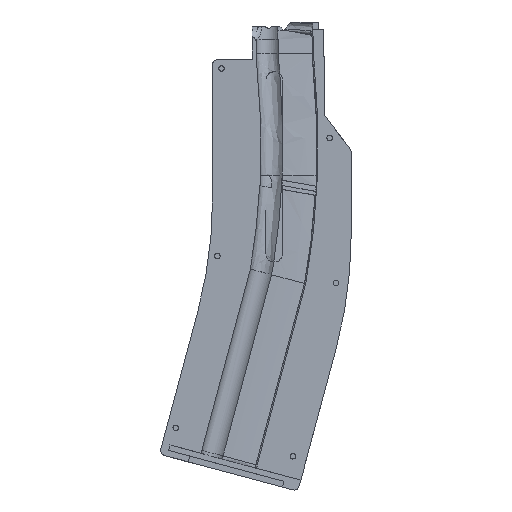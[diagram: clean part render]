
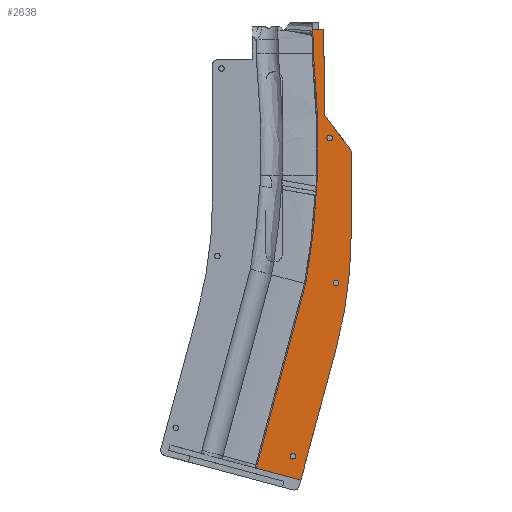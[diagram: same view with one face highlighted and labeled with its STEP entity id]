
A CAD part, front view. The second image highlights one B-rep face of the part: STEP entity #2638.
In plain terms, the highlighted planar face has unit normal (0, -1, 0).
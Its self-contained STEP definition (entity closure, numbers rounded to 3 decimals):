
#15=FACE_BOUND('',#458,.T.);
#16=FACE_BOUND('',#459,.T.);
#17=FACE_BOUND('',#460,.T.);
#39=PLANE('',#2853);
#101=B_SPLINE_CURVE_WITH_KNOTS('',3,(#4024,#4025,#4026,#4027),
 .UNSPECIFIED.,.F.,.F.,(4,4),(-10.66,-5.148),
 .UNSPECIFIED.);
#102=B_SPLINE_CURVE_WITH_KNOTS('',3,(#4029,#4030,#4031,#4032),
 .UNSPECIFIED.,.F.,.F.,(4,4),(-5.148,-0.178),
 .UNSPECIFIED.);
#290=FACE_OUTER_BOUND('',#457,.T.);
#457=EDGE_LOOP('',(#1914,#1915,#1916,#1917,#1918,#1919,#1920,#1921,#1922,
#1923,#1924,#1925,#1926,#1927,#1928,#1929,#1930,#1931,#1932));
#458=EDGE_LOOP('',(#1933));
#459=EDGE_LOOP('',(#1934));
#460=EDGE_LOOP('',(#1935));
#638=CIRCLE('',#2803,3.);
#660=CIRCLE('',#2848,200.);
#662=CIRCLE('',#2851,2.5);
#663=CIRCLE('',#2854,2.);
#664=CIRCLE('',#2855,318.391);
#665=CIRCLE('',#2856,1.25);
#666=CIRCLE('',#2857,1.25);
#667=CIRCLE('',#2858,1.25);
#745=LINE('',#3823,#918);
#759=LINE('',#3877,#932);
#761=LINE('',#3881,#934);
#764=LINE('',#3893,#937);
#782=LINE('',#3943,#955);
#786=LINE('',#3957,#959);
#789=LINE('',#4014,#962);
#790=LINE('',#4016,#963);
#791=LINE('',#4018,#964);
#792=LINE('',#4022,#965);
#793=LINE('',#4034,#966);
#794=LINE('',#4036,#967);
#918=VECTOR('',#3109,10.);
#932=VECTOR('',#3151,10.);
#934=VECTOR('',#3155,10.);
#937=VECTOR('',#3170,10.);
#955=VECTOR('',#3218,10.);
#959=VECTOR('',#3234,10.);
#962=VECTOR('',#3239,10.);
#963=VECTOR('',#3240,10.);
#964=VECTOR('',#3241,10.);
#965=VECTOR('',#3244,10.);
#966=VECTOR('',#3245,10.);
#967=VECTOR('',#3246,10.);
#1088=VERTEX_POINT('',#3800);
#1089=VERTEX_POINT('',#3802);
#1094=VERTEX_POINT('',#3821);
#1111=VERTEX_POINT('',#3875);
#1112=VERTEX_POINT('',#3879);
#1115=VERTEX_POINT('',#3892);
#1131=VERTEX_POINT('',#3940);
#1132=VERTEX_POINT('',#3942);
#1135=VERTEX_POINT('',#3952);
#1136=VERTEX_POINT('',#3956);
#1143=VERTEX_POINT('',#4013);
#1144=VERTEX_POINT('',#4015);
#1145=VERTEX_POINT('',#4017);
#1146=VERTEX_POINT('',#4019);
#1147=VERTEX_POINT('',#4021);
#1148=VERTEX_POINT('',#4023);
#1149=VERTEX_POINT('',#4028);
#1150=VERTEX_POINT('',#4033);
#1151=VERTEX_POINT('',#4035);
#1152=VERTEX_POINT('',#4038);
#1153=VERTEX_POINT('',#4040);
#1154=VERTEX_POINT('',#4042);
#1350=EDGE_CURVE('',#1088,#1089,#638,.T.);
#1361=EDGE_CURVE('',#1088,#1094,#745,.T.);
#1384=EDGE_CURVE('',#1094,#1111,#759,.T.);
#1386=EDGE_CURVE('',#1111,#1112,#761,.T.);
#1391=EDGE_CURVE('',#1115,#1089,#764,.T.);
#1416=EDGE_CURVE('',#1132,#1131,#782,.T.);
#1418=EDGE_CURVE('',#1115,#1131,#660,.T.);
#1422=EDGE_CURVE('',#1135,#1112,#662,.T.);
#1423=EDGE_CURVE('',#1132,#1136,#786,.T.);
#1431=EDGE_CURVE('',#1143,#1135,#789,.T.);
#1432=EDGE_CURVE('',#1143,#1144,#790,.T.);
#1433=EDGE_CURVE('',#1144,#1145,#791,.T.);
#1434=EDGE_CURVE('',#1145,#1146,#663,.T.);
#1435=EDGE_CURVE('',#1146,#1147,#792,.T.);
#1436=EDGE_CURVE('',#1147,#1148,#101,.T.);
#1437=EDGE_CURVE('',#1148,#1149,#102,.T.);
#1438=EDGE_CURVE('',#1149,#1150,#793,.T.);
#1439=EDGE_CURVE('',#1150,#1151,#794,.T.);
#1440=EDGE_CURVE('',#1151,#1136,#664,.T.);
#1441=EDGE_CURVE('',#1152,#1152,#665,.T.);
#1442=EDGE_CURVE('',#1153,#1153,#666,.T.);
#1443=EDGE_CURVE('',#1154,#1154,#667,.T.);
#1914=ORIENTED_EDGE('',*,*,#1350,.F.);
#1915=ORIENTED_EDGE('',*,*,#1361,.T.);
#1916=ORIENTED_EDGE('',*,*,#1384,.T.);
#1917=ORIENTED_EDGE('',*,*,#1386,.T.);
#1918=ORIENTED_EDGE('',*,*,#1422,.F.);
#1919=ORIENTED_EDGE('',*,*,#1431,.F.);
#1920=ORIENTED_EDGE('',*,*,#1432,.T.);
#1921=ORIENTED_EDGE('',*,*,#1433,.T.);
#1922=ORIENTED_EDGE('',*,*,#1434,.T.);
#1923=ORIENTED_EDGE('',*,*,#1435,.T.);
#1924=ORIENTED_EDGE('',*,*,#1436,.T.);
#1925=ORIENTED_EDGE('',*,*,#1437,.T.);
#1926=ORIENTED_EDGE('',*,*,#1438,.T.);
#1927=ORIENTED_EDGE('',*,*,#1439,.T.);
#1928=ORIENTED_EDGE('',*,*,#1440,.T.);
#1929=ORIENTED_EDGE('',*,*,#1423,.F.);
#1930=ORIENTED_EDGE('',*,*,#1416,.T.);
#1931=ORIENTED_EDGE('',*,*,#1418,.F.);
#1932=ORIENTED_EDGE('',*,*,#1391,.T.);
#1933=ORIENTED_EDGE('',*,*,#1441,.T.);
#1934=ORIENTED_EDGE('',*,*,#1442,.T.);
#1935=ORIENTED_EDGE('',*,*,#1443,.T.);
#2638=ADVANCED_FACE('',(#290,#15,#16,#17),#39,.T.);
#2803=AXIS2_PLACEMENT_3D('',#3803,#3086,#3087);
#2848=AXIS2_PLACEMENT_3D('',#3946,#3222,#3223);
#2851=AXIS2_PLACEMENT_3D('',#3954,#3230,#3231);
#2853=AXIS2_PLACEMENT_3D('',#4012,#3237,#3238);
#2854=AXIS2_PLACEMENT_3D('',#4020,#3242,#3243);
#2855=AXIS2_PLACEMENT_3D('',#4037,#3247,#3248);
#2856=AXIS2_PLACEMENT_3D('',#4039,#3249,#3250);
#2857=AXIS2_PLACEMENT_3D('',#4041,#3251,#3252);
#2858=AXIS2_PLACEMENT_3D('',#4043,#3253,#3254);
#3086=DIRECTION('center_axis',(0.,1.,0.));
#3087=DIRECTION('ref_axis',(0.947,0.,0.322));
#3109=DIRECTION('',(-0.61,0.,0.792));
#3151=DIRECTION('',(0.792,0.,0.61));
#3155=DIRECTION('',(0.,0.,1.));
#3170=DIRECTION('',(0.,0.,1.));
#3218=DIRECTION('',(0.259,0.,0.966));
#3222=DIRECTION('center_axis',(0.,1.,0.));
#3223=DIRECTION('ref_axis',(0.991,0.,-0.131));
#3230=DIRECTION('center_axis',(0.,1.,0.));
#3231=DIRECTION('ref_axis',(0.707,0.,0.707));
#3234=DIRECTION('',(-0.966,0.,0.259));
#3237=DIRECTION('center_axis',(0.,-1.,0.));
#3238=DIRECTION('ref_axis',(1.,0.,0.));
#3239=DIRECTION('',(0.,0.,-1.));
#3240=DIRECTION('',(-1.,0.,0.));
#3241=DIRECTION('',(0.,0.,-1.));
#3242=DIRECTION('center_axis',(0.,1.,0.));
#3243=DIRECTION('ref_axis',(0.77,0.,0.639));
#3244=DIRECTION('',(0.,0.,-1.));
#3245=DIRECTION('',(-0.259,0.,-0.966));
#3246=DIRECTION('',(-0.966,0.,0.259));
#3247=DIRECTION('center_axis',(0.,1.,0.));
#3248=DIRECTION('ref_axis',(0.983,0.,-0.185));
#3249=DIRECTION('center_axis',(0.,1.,0.));
#3250=DIRECTION('ref_axis',(0.,0.,-1.));
#3251=DIRECTION('center_axis',(0.,1.,0.));
#3252=DIRECTION('ref_axis',(0.,0.,-1.));
#3253=DIRECTION('center_axis',(0.,1.,0.));
#3254=DIRECTION('ref_axis',(0.,0.,-1.));
#3800=CARTESIAN_POINT('',(908.25,-16.727,-9.367));
#3802=CARTESIAN_POINT('',(908.874,-16.727,-11.198));
#3803=CARTESIAN_POINT('Origin',(905.874,-16.727,-11.198));
#3821=CARTESIAN_POINT('',(896.848,-16.727,5.44));
#3823=CARTESIAN_POINT('',(908.474,-16.727,-9.657));
#3875=CARTESIAN_POINT('',(896.854,-16.727,5.444));
#3877=CARTESIAN_POINT('',(894.623,-16.727,3.726));
#3879=CARTESIAN_POINT('',(896.854,-16.727,30.987));
#3881=CARTESIAN_POINT('',(896.854,-16.727,9.155));
#3892=CARTESIAN_POINT('',(908.874,-16.727,-48.17));
#3893=CARTESIAN_POINT('',(908.874,-16.727,-9.489));
#3940=CARTESIAN_POINT('',(902.059,-16.727,-99.934));
#3942=CARTESIAN_POINT('',(886.076,-16.727,-159.581));
#3943=CARTESIAN_POINT('',(905.041,-16.727,-88.804));
#3946=CARTESIAN_POINT('Origin',(708.874,-16.727,-48.17));
#3952=CARTESIAN_POINT('',(896.124,-16.727,32.752));
#3954=CARTESIAN_POINT('Origin',(894.354,-16.727,30.987));
#3956=CARTESIAN_POINT('',(866.031,-16.727,-154.21));
#3957=CARTESIAN_POINT('',(861.108,-16.727,-152.891));
#4012=CARTESIAN_POINT('Origin',(903.624,-16.727,-12.565));
#4013=CARTESIAN_POINT('',(896.124,-16.727,44.387));
#4014=CARTESIAN_POINT('',(896.124,-16.727,-42.694));
#4015=CARTESIAN_POINT('',(891.532,-16.727,44.387));
#4016=CARTESIAN_POINT('',(884.621,-16.727,44.387));
#4017=CARTESIAN_POINT('',(891.532,-16.727,41.603));
#4018=CARTESIAN_POINT('',(891.532,-16.727,14.476));
#4019=CARTESIAN_POINT('',(891.804,-16.727,40.597));
#4020=CARTESIAN_POINT('Origin',(889.804,-16.727,40.597));
#4021=CARTESIAN_POINT('',(891.804,-16.727,33.487));
#4022=CARTESIAN_POINT('',(891.804,-16.727,12.411));
#4023=CARTESIAN_POINT('',(893.588,-16.727,-21.513));
#4024=CARTESIAN_POINT('Ctrl Pts',(891.804,-16.727,33.487));
#4025=CARTESIAN_POINT('Ctrl Pts',(893.616,-16.727,14.51));
#4026=CARTESIAN_POINT('Ctrl Pts',(894.224,-16.727,-3.789));
#4027=CARTESIAN_POINT('Ctrl Pts',(893.588,-16.727,-21.513));
#4028=CARTESIAN_POINT('',(888.307,-16.727,-70.728));
#4029=CARTESIAN_POINT('Ctrl Pts',(893.588,-16.727,-21.513));
#4030=CARTESIAN_POINT('Ctrl Pts',(892.983,-16.727,-38.366));
#4031=CARTESIAN_POINT('Ctrl Pts',(891.251,-16.727,-54.706));
#4032=CARTESIAN_POINT('Ctrl Pts',(888.307,-16.727,-70.728));
#4033=CARTESIAN_POINT('',(866.334,-16.727,-152.735));
#4034=CARTESIAN_POINT('',(888.307,-16.727,-70.728));
#4035=CARTESIAN_POINT('',(866.307,-16.727,-152.728));
#4036=CARTESIAN_POINT('',(842.596,-16.727,-146.375));
#4037=CARTESIAN_POINT('Origin',(553.158,-16.727,-95.196));
#4038=CARTESIAN_POINT('',(899.124,-16.727,-3.375));
#4039=CARTESIAN_POINT('Origin',(899.124,-16.727,-4.625));
#4040=CARTESIAN_POINT('',(882.493,-16.727,-147.557));
#4041=CARTESIAN_POINT('Origin',(882.493,-16.727,-148.807));
#4042=CARTESIAN_POINT('',(901.936,-16.727,-69.081));
#4043=CARTESIAN_POINT('Origin',(901.936,-16.727,-70.331));
